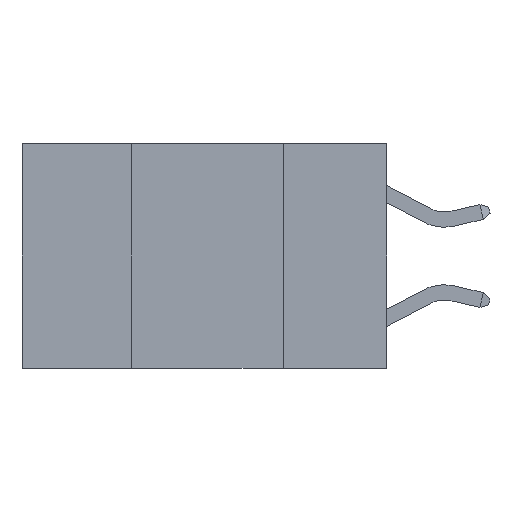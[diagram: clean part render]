
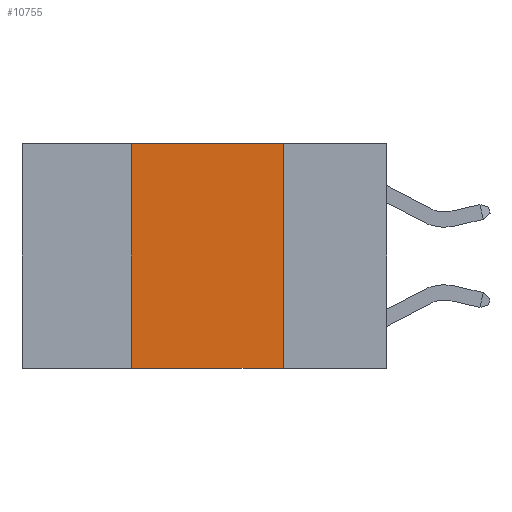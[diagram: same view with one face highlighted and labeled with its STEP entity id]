
A CAD part, left-side view. The second image highlights one B-rep face of the part: STEP entity #10755.
In plain terms, the highlighted planar face has unit normal (-1, 0, 0).
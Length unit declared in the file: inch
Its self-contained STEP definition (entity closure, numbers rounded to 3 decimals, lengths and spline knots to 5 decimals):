
#611 = LINE ( 'NONE', #10813, #11705 ) ;
#2051 = LINE ( 'NONE', #18597, #17615 ) ;
#2349 = PLANE ( 'NONE',  #10596 ) ;
#2924 = CARTESIAN_POINT ( 'NONE',  ( 0., 0.17, -0.37 ) ) ;
#3706 = ORIENTED_EDGE ( 'NONE', *, *, #7832, .F. ) ;
#3732 = CARTESIAN_POINT ( 'NONE',  ( 0., 0.42, 0. ) ) ;
#4173 = ORIENTED_EDGE ( 'NONE', *, *, #11253, .T. ) ;
#4680 = DIRECTION ( 'NONE',  ( 0., -1., 0. ) ) ;
#5690 = VERTEX_POINT ( 'NONE', #11834 ) ;
#5795 = VECTOR ( 'NONE', #15804, 39.37008 ) ;
#5984 = CARTESIAN_POINT ( 'NONE',  ( 0., 0.42, 0. ) ) ;
#6312 = VECTOR ( 'NONE', #12790, 39.37008 ) ;
#6631 = DIRECTION ( 'NONE',  ( 0., -1., 0. ) ) ;
#6983 = DIRECTION ( 'NONE',  ( 1., 0., 0. ) ) ;
#6997 = VERTEX_POINT ( 'NONE', #5984 ) ;
#7231 = ORIENTED_EDGE ( 'NONE', *, *, #14922, .F. ) ;
#7832 = EDGE_CURVE ( 'NONE', #5690, #6997, #18788, .T. ) ;
#10596 = AXIS2_PLACEMENT_3D ( 'NONE', #12986, #6983, #17530 ) ;
#10755 = ADVANCED_FACE ( 'NONE', ( #14585 ), #2349, .F. ) ;
#10813 = CARTESIAN_POINT ( 'NONE',  ( 0., 0.6, 0. ) ) ;
#11253 = EDGE_CURVE ( 'NONE', #5690, #16507, #2051, .T. ) ;
#11705 = VECTOR ( 'NONE', #4680, 39.37008 ) ;
#11834 = CARTESIAN_POINT ( 'NONE',  ( 0., 0.42, -0.37 ) ) ;
#12790 = DIRECTION ( 'NONE',  ( 0., 0., 1. ) ) ;
#12986 = CARTESIAN_POINT ( 'NONE',  ( 0., 0.6, 0. ) ) ;
#14282 = CARTESIAN_POINT ( 'NONE',  ( 0., 0.17, 0. ) ) ;
#14585 = FACE_OUTER_BOUND ( 'NONE', #19291, .T. ) ;
#14922 = EDGE_CURVE ( 'NONE', #18082, #16507, #17826, .T. ) ;
#15299 = ORIENTED_EDGE ( 'NONE', *, *, #15962, .F. ) ;
#15804 = DIRECTION ( 'NONE',  ( 0., 0., -1. ) ) ;
#15962 = EDGE_CURVE ( 'NONE', #6997, #18082, #611, .T. ) ;
#16507 = VERTEX_POINT ( 'NONE', #2924 ) ;
#17530 = DIRECTION ( 'NONE',  ( 0., 0., -1. ) ) ;
#17615 = VECTOR ( 'NONE', #6631, 39.37008 ) ;
#17826 = LINE ( 'NONE', #14282, #5795 ) ;
#18082 = VERTEX_POINT ( 'NONE', #18534 ) ;
#18534 = CARTESIAN_POINT ( 'NONE',  ( 0., 0.17, 0. ) ) ;
#18597 = CARTESIAN_POINT ( 'NONE',  ( 0., 0.6, -0.37 ) ) ;
#18788 = LINE ( 'NONE', #3732, #6312 ) ;
#19291 = EDGE_LOOP ( 'NONE', ( #7231, #15299, #3706, #4173 ) ) ;
